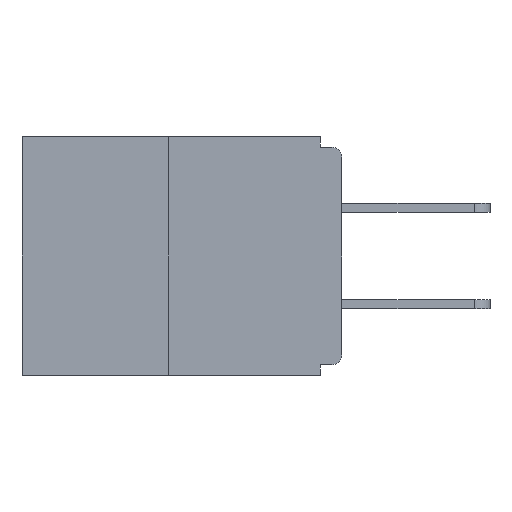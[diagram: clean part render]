
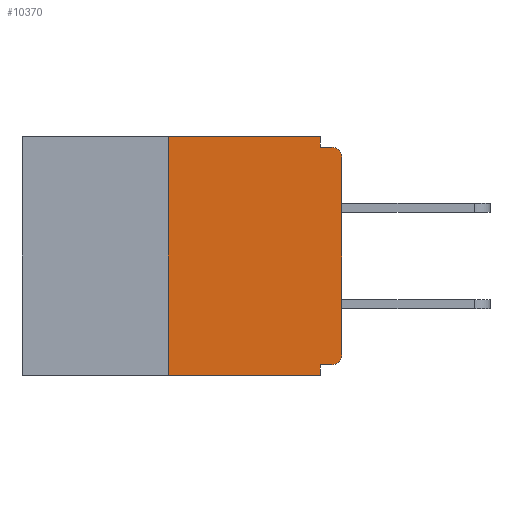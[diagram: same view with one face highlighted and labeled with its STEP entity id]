
A CAD part, left-side view. The second image highlights one B-rep face of the part: STEP entity #10370.
In plain terms, the highlighted planar face has unit normal (-1, 0, 0).
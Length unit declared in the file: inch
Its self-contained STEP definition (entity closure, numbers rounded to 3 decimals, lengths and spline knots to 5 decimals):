
#343 = EDGE_LOOP ( 'NONE', ( #9557, #2466, #12559, #20846, #2839, #8297, #6162, #20761, #18308, #4637 ) ) ;
#515 = CARTESIAN_POINT ( 'NONE',  ( 0., 0.031, -0.328 ) ) ;
#963 = VERTEX_POINT ( 'NONE', #5244 ) ;
#1011 = LINE ( 'NONE', #6092, #13183 ) ;
#2466 = ORIENTED_EDGE ( 'NONE', *, *, #13563, .F. ) ;
#2614 = VECTOR ( 'NONE', #5821, 39.37008 ) ;
#2839 = ORIENTED_EDGE ( 'NONE', *, *, #12096, .F. ) ;
#2858 = EDGE_CURVE ( 'NONE', #12493, #22802, #18767, .T. ) ;
#3645 = VECTOR ( 'NONE', #19826, 39.37008 ) ;
#3648 = AXIS2_PLACEMENT_3D ( 'NONE', #5922, #6077, #22370 ) ;
#3832 = VERTEX_POINT ( 'NONE', #14805 ) ;
#4446 = LINE ( 'NONE', #16542, #5306 ) ;
#4603 = VERTEX_POINT ( 'NONE', #20222 ) ;
#4637 = ORIENTED_EDGE ( 'NONE', *, *, #8831, .F. ) ;
#4808 = VECTOR ( 'NONE', #14140, 39.37008 ) ;
#4859 = CIRCLE ( 'NONE', #3648, 0.015 ) ;
#5002 = DIRECTION ( 'NONE',  ( 1., 0., 0. ) ) ;
#5244 = CARTESIAN_POINT ( 'NONE',  ( 0., 0., -0.313 ) ) ;
#5306 = VECTOR ( 'NONE', #7495, 39.37008 ) ;
#5626 = VECTOR ( 'NONE', #17138, 39.37008 ) ;
#5821 = DIRECTION ( 'NONE',  ( 0., -1., 0. ) ) ;
#5922 = CARTESIAN_POINT ( 'NONE',  ( 0., 0.015, -0.313 ) ) ;
#6077 = DIRECTION ( 'NONE',  ( -1., 0., 0. ) ) ;
#6092 = CARTESIAN_POINT ( 'NONE',  ( 0., 0.25, 0. ) ) ;
#6162 = ORIENTED_EDGE ( 'NONE', *, *, #16915, .T. ) ;
#6816 = DIRECTION ( 'NONE',  ( 0., 0., -1. ) ) ;
#6868 = AXIS2_PLACEMENT_3D ( 'NONE', #22894, #5002, #6816 ) ;
#7348 = VERTEX_POINT ( 'NONE', #17801 ) ;
#7495 = DIRECTION ( 'NONE',  ( 0., 0., -1. ) ) ;
#7653 = VERTEX_POINT ( 'NONE', #515 ) ;
#8139 = CARTESIAN_POINT ( 'NONE',  ( 0., 0., 0. ) ) ;
#8297 = ORIENTED_EDGE ( 'NONE', *, *, #16335, .T. ) ;
#8319 = CARTESIAN_POINT ( 'NONE',  ( 0., 0.25, 0. ) ) ;
#8656 = CARTESIAN_POINT ( 'NONE',  ( 0., 0., -0.328 ) ) ;
#8831 = EDGE_CURVE ( 'NONE', #22802, #3832, #9567, .T. ) ;
#9557 = ORIENTED_EDGE ( 'NONE', *, *, #2858, .F. ) ;
#9567 = LINE ( 'NONE', #21176, #4808 ) ;
#10070 = LINE ( 'NONE', #11943, #5626 ) ;
#10078 = DIRECTION ( 'NONE',  ( 0., 0., 1. ) ) ;
#10370 = ADVANCED_FACE ( 'NONE', ( #14090 ), #15698, .F. ) ;
#10759 = VERTEX_POINT ( 'NONE', #15004 ) ;
#10791 = CARTESIAN_POINT ( 'NONE',  ( 0., 0., -0.03 ) ) ;
#11747 = AXIS2_PLACEMENT_3D ( 'NONE', #22397, #15201, #22962 ) ;
#11943 = CARTESIAN_POINT ( 'NONE',  ( 0., 0., -0.015 ) ) ;
#12096 = EDGE_CURVE ( 'NONE', #10759, #7653, #15841, .T. ) ;
#12493 = VERTEX_POINT ( 'NONE', #8319 ) ;
#12559 = ORIENTED_EDGE ( 'NONE', *, *, #13982, .T. ) ;
#12575 = EDGE_CURVE ( 'NONE', #3832, #4603, #10070, .T. ) ;
#12836 = CARTESIAN_POINT ( 'NONE',  ( 0., 0.46, -0.343 ) ) ;
#12935 = DIRECTION ( 'NONE',  ( 0., 0., 1. ) ) ;
#13015 = VECTOR ( 'NONE', #10078, 39.37008 ) ;
#13159 = LINE ( 'NONE', #12836, #23122 ) ;
#13183 = VECTOR ( 'NONE', #12935, 39.37008 ) ;
#13442 = EDGE_CURVE ( 'NONE', #7653, #7348, #4446, .T. ) ;
#13563 = EDGE_CURVE ( 'NONE', #22367, #12493, #1011, .T. ) ;
#13968 = CIRCLE ( 'NONE', #11747, 0.015 ) ;
#13982 = EDGE_CURVE ( 'NONE', #22367, #7348, #13159, .T. ) ;
#14090 = FACE_OUTER_BOUND ( 'NONE', #343, .T. ) ;
#14140 = DIRECTION ( 'NONE',  ( 0., 0., -1. ) ) ;
#14805 = CARTESIAN_POINT ( 'NONE',  ( 0., 0.031, -0.015 ) ) ;
#15004 = CARTESIAN_POINT ( 'NONE',  ( 0., 0.015, -0.328 ) ) ;
#15201 = DIRECTION ( 'NONE',  ( -1., 0., 0. ) ) ;
#15293 = EDGE_CURVE ( 'NONE', #18273, #4603, #13968, .T. ) ;
#15698 = PLANE ( 'NONE',  #6868 ) ;
#15841 = LINE ( 'NONE', #8656, #3645 ) ;
#16275 = CARTESIAN_POINT ( 'NONE',  ( 0., 0.46, 0. ) ) ;
#16335 = EDGE_CURVE ( 'NONE', #10759, #963, #4859, .T. ) ;
#16514 = DIRECTION ( 'NONE',  ( 0., -1., 0. ) ) ;
#16542 = CARTESIAN_POINT ( 'NONE',  ( 0., 0.031, -0.343 ) ) ;
#16915 = EDGE_CURVE ( 'NONE', #963, #18273, #17875, .T. ) ;
#17138 = DIRECTION ( 'NONE',  ( 0., -1., 0. ) ) ;
#17801 = CARTESIAN_POINT ( 'NONE',  ( 0., 0.031, -0.343 ) ) ;
#17875 = LINE ( 'NONE', #8139, #13015 ) ;
#18273 = VERTEX_POINT ( 'NONE', #10791 ) ;
#18308 = ORIENTED_EDGE ( 'NONE', *, *, #12575, .F. ) ;
#18767 = LINE ( 'NONE', #16275, #2614 ) ;
#19826 = DIRECTION ( 'NONE',  ( 0., 1., 0. ) ) ;
#20222 = CARTESIAN_POINT ( 'NONE',  ( 0., 0.015, -0.015 ) ) ;
#20428 = CARTESIAN_POINT ( 'NONE',  ( 0., 0.031, 0. ) ) ;
#20761 = ORIENTED_EDGE ( 'NONE', *, *, #15293, .T. ) ;
#20846 = ORIENTED_EDGE ( 'NONE', *, *, #13442, .F. ) ;
#21176 = CARTESIAN_POINT ( 'NONE',  ( 0., 0.031, 0. ) ) ;
#21587 = CARTESIAN_POINT ( 'NONE',  ( 0., 0.25, -0.343 ) ) ;
#22367 = VERTEX_POINT ( 'NONE', #21587 ) ;
#22370 = DIRECTION ( 'NONE',  ( 0., 0., -1. ) ) ;
#22397 = CARTESIAN_POINT ( 'NONE',  ( 0., 0.015, -0.03 ) ) ;
#22802 = VERTEX_POINT ( 'NONE', #20428 ) ;
#22894 = CARTESIAN_POINT ( 'NONE',  ( 0., 0.46, 0. ) ) ;
#22962 = DIRECTION ( 'NONE',  ( 0., 0., -1. ) ) ;
#23122 = VECTOR ( 'NONE', #16514, 39.37008 ) ;
